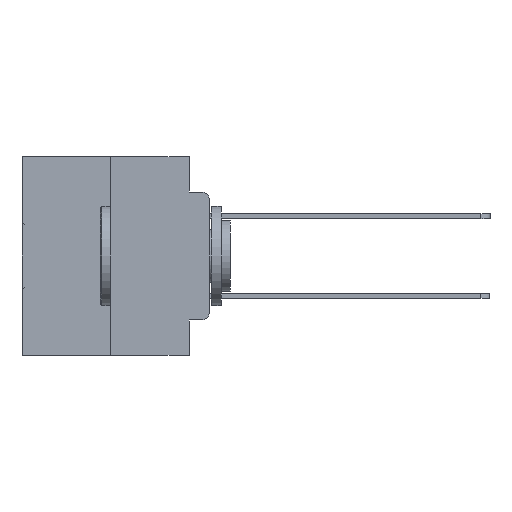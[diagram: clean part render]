
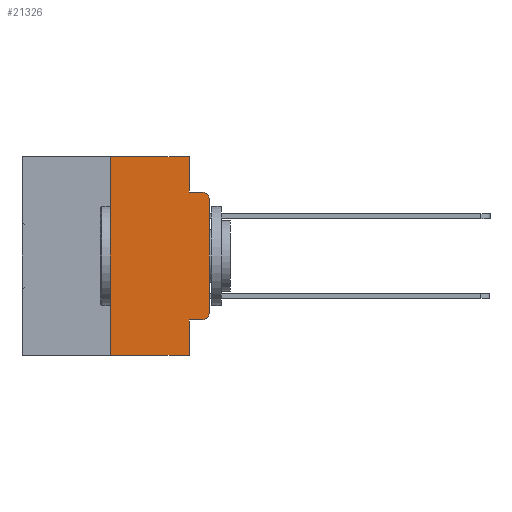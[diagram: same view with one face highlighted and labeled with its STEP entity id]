
A CAD part, left-side view. The second image highlights one B-rep face of the part: STEP entity #21326.
In plain terms, the highlighted planar face has unit normal (-1, 0, 0).
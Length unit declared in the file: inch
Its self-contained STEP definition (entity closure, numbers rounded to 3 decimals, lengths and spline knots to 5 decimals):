
#274 = CIRCLE ( 'NONE', #586, 0.02 ) ;
#320 = EDGE_CURVE ( 'NONE', #26843, #28672, #11637, .T. ) ;
#383 = CARTESIAN_POINT ( 'NONE',  ( 0., 0.25, -0.5 ) ) ;
#426 = CARTESIAN_POINT ( 'NONE',  ( 0., 0.473, 0. ) ) ;
#586 = AXIS2_PLACEMENT_3D ( 'NONE', #21708, #5839, #24340 ) ;
#1472 = EDGE_CURVE ( 'NONE', #28672, #29294, #24270, .T. ) ;
#2302 = ORIENTED_EDGE ( 'NONE', *, *, #13815, .T. ) ;
#2310 = VERTEX_POINT ( 'NONE', #27879 ) ;
#2503 = DIRECTION ( 'NONE',  ( -1., 0., 0. ) ) ;
#3062 = CARTESIAN_POINT ( 'NONE',  ( 0., 0.051, -0.0885 ) ) ;
#3222 = DIRECTION ( 'NONE',  ( 1., 0., 0. ) ) ;
#3974 = ORIENTED_EDGE ( 'NONE', *, *, #30312, .T. ) ;
#4216 = EDGE_CURVE ( 'NONE', #28076, #21913, #15075, .T. ) ;
#5199 = VERTEX_POINT ( 'NONE', #13055 ) ;
#5821 = CARTESIAN_POINT ( 'NONE',  ( 0., 0.473, 0. ) ) ;
#5839 = DIRECTION ( 'NONE',  ( -1., 0., 0. ) ) ;
#6555 = CARTESIAN_POINT ( 'NONE',  ( 0., 0.25, 0. ) ) ;
#6865 = LINE ( 'NONE', #26337, #20076 ) ;
#7214 = VECTOR ( 'NONE', #28561, 39.37008 ) ;
#7844 = ORIENTED_EDGE ( 'NONE', *, *, #23663, .T. ) ;
#8578 = DIRECTION ( 'NONE',  ( 0., -1., 0. ) ) ;
#8695 = DIRECTION ( 'NONE',  ( 0., 0., -1. ) ) ;
#8813 = CARTESIAN_POINT ( 'NONE',  ( 0., 0.051, 0. ) ) ;
#9390 = DIRECTION ( 'NONE',  ( 0., 0., 1. ) ) ;
#11126 = EDGE_CURVE ( 'NONE', #11817, #14987, #6865, .T. ) ;
#11637 = LINE ( 'NONE', #426, #31752 ) ;
#11817 = VERTEX_POINT ( 'NONE', #31722 ) ;
#12081 = VECTOR ( 'NONE', #9390, 39.37008 ) ;
#12420 = DIRECTION ( 'NONE',  ( 0., -1., 0. ) ) ;
#12855 = DIRECTION ( 'NONE',  ( 0., 0., -1. ) ) ;
#12875 = VECTOR ( 'NONE', #12420, 39.37008 ) ;
#13055 = CARTESIAN_POINT ( 'NONE',  ( 0., 0.02, -0.0885 ) ) ;
#13702 = LINE ( 'NONE', #15044, #12875 ) ;
#13766 = PLANE ( 'NONE',  #17465 ) ;
#13815 = EDGE_CURVE ( 'NONE', #25273, #2310, #19028, .T. ) ;
#14987 = VERTEX_POINT ( 'NONE', #29861 ) ;
#15044 = CARTESIAN_POINT ( 'NONE',  ( 0., 0.051, -0.0885 ) ) ;
#15075 = LINE ( 'NONE', #21738, #7214 ) ;
#15243 = ORIENTED_EDGE ( 'NONE', *, *, #30493, .F. ) ;
#17465 = AXIS2_PLACEMENT_3D ( 'NONE', #5821, #3222, #21796 ) ;
#18430 = CARTESIAN_POINT ( 'NONE',  ( 0., 0.02, -0.3915 ) ) ;
#19028 = LINE ( 'NONE', #30398, #12081 ) ;
#19232 = CARTESIAN_POINT ( 'NONE',  ( 0., 0., -0.3915 ) ) ;
#19358 = ORIENTED_EDGE ( 'NONE', *, *, #19928, .F. ) ;
#19640 = VECTOR ( 'NONE', #12855, 39.37008 ) ;
#19928 = EDGE_CURVE ( 'NONE', #11817, #21913, #25804, .T. ) ;
#20076 = VECTOR ( 'NONE', #23735, 39.37008 ) ;
#20419 = CARTESIAN_POINT ( 'NONE',  ( 0., 0.25, 0. ) ) ;
#21082 = DIRECTION ( 'NONE',  ( 0., 0., -1. ) ) ;
#21326 = ADVANCED_FACE ( 'NONE', ( #24892 ), #13766, .F. ) ;
#21708 = CARTESIAN_POINT ( 'NONE',  ( 0., 0.02, -0.1085 ) ) ;
#21738 = CARTESIAN_POINT ( 'NONE',  ( 0., 0.473, -0.5 ) ) ;
#21796 = DIRECTION ( 'NONE',  ( 0., 0., -1. ) ) ;
#21913 = VERTEX_POINT ( 'NONE', #29917 ) ;
#22811 = EDGE_CURVE ( 'NONE', #29294, #5199, #13702, .T. ) ;
#23663 = EDGE_CURVE ( 'NONE', #14987, #25273, #28428, .T. ) ;
#23735 = DIRECTION ( 'NONE',  ( 0., -1., 0. ) ) ;
#24270 = LINE ( 'NONE', #8813, #32079 ) ;
#24340 = DIRECTION ( 'NONE',  ( 0., 0., -1. ) ) ;
#24892 = FACE_OUTER_BOUND ( 'NONE', #33409, .T. ) ;
#25273 = VERTEX_POINT ( 'NONE', #19232 ) ;
#25804 = LINE ( 'NONE', #28577, #19640 ) ;
#25918 = ORIENTED_EDGE ( 'NONE', *, *, #1472, .F. ) ;
#26337 = CARTESIAN_POINT ( 'NONE',  ( 0., 0.051, -0.4115 ) ) ;
#26843 = VERTEX_POINT ( 'NONE', #20419 ) ;
#27879 = CARTESIAN_POINT ( 'NONE',  ( 0., 0., -0.1085 ) ) ;
#28076 = VERTEX_POINT ( 'NONE', #383 ) ;
#28428 = CIRCLE ( 'NONE', #32238, 0.02 ) ;
#28561 = DIRECTION ( 'NONE',  ( 0., -1., 0. ) ) ;
#28577 = CARTESIAN_POINT ( 'NONE',  ( 0., 0.051, 0. ) ) ;
#28672 = VERTEX_POINT ( 'NONE', #31884 ) ;
#28808 = VECTOR ( 'NONE', #32922, 39.37008 ) ;
#29294 = VERTEX_POINT ( 'NONE', #3062 ) ;
#29636 = LINE ( 'NONE', #6555, #28808 ) ;
#29861 = CARTESIAN_POINT ( 'NONE',  ( 0., 0.02, -0.4115 ) ) ;
#29917 = CARTESIAN_POINT ( 'NONE',  ( 0., 0.051, -0.5 ) ) ;
#30312 = EDGE_CURVE ( 'NONE', #2310, #5199, #274, .T. ) ;
#30398 = CARTESIAN_POINT ( 'NONE',  ( 0., 0., 0. ) ) ;
#30493 = EDGE_CURVE ( 'NONE', #28076, #26843, #29636, .T. ) ;
#31722 = CARTESIAN_POINT ( 'NONE',  ( 0., 0.051, -0.4115 ) ) ;
#31752 = VECTOR ( 'NONE', #8578, 39.37008 ) ;
#31884 = CARTESIAN_POINT ( 'NONE',  ( 0., 0.051, 0. ) ) ;
#32079 = VECTOR ( 'NONE', #8695, 39.37008 ) ;
#32091 = ORIENTED_EDGE ( 'NONE', *, *, #22811, .F. ) ;
#32238 = AXIS2_PLACEMENT_3D ( 'NONE', #18430, #2503, #21082 ) ;
#32512 = ORIENTED_EDGE ( 'NONE', *, *, #4216, .T. ) ;
#32922 = DIRECTION ( 'NONE',  ( 0., 0., 1. ) ) ;
#33409 = EDGE_LOOP ( 'NONE', ( #2302, #3974, #32091, #25918, #33698, #15243, #32512, #19358, #34101, #7844 ) ) ;
#33698 = ORIENTED_EDGE ( 'NONE', *, *, #320, .F. ) ;
#34101 = ORIENTED_EDGE ( 'NONE', *, *, #11126, .T. ) ;
